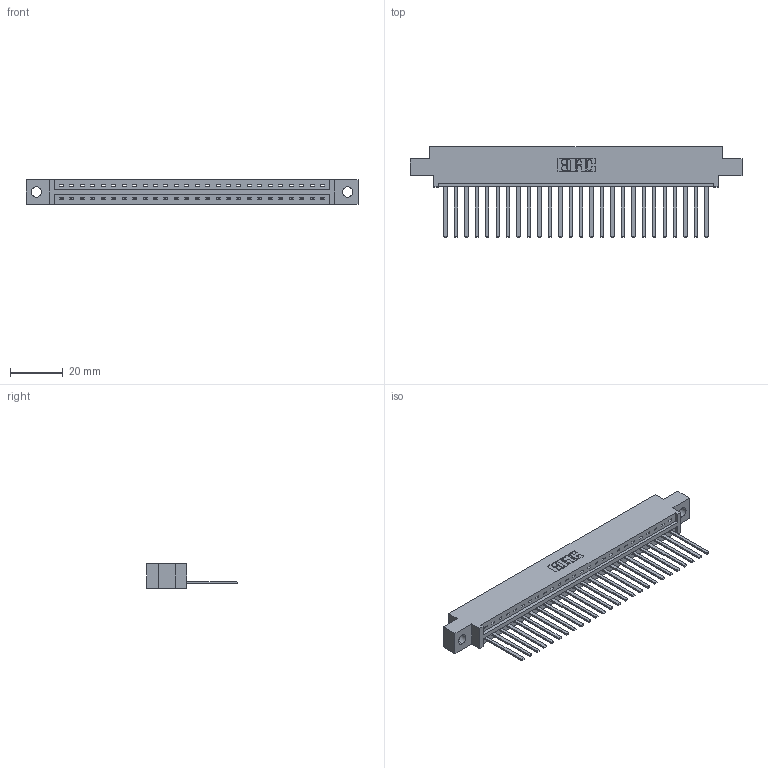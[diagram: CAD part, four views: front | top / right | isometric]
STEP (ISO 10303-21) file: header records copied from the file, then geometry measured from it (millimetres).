
FILE_DESCRIPTION (( 'STEP AP203' ), '1' );
FILE_NAME ('337-026-544-604.STEP', '2019-09-30T19:03:22', ( '' ), ( '' ), 'SwSTEP 2.0', 'SolidWorks 2016', '' );
FILE_SCHEMA (( 'CONFIG_CONTROL_DESIGN' ));
Length unit declared in the file: inch
Products named in the file (3): 337-026-544-604; 345-292-001_345-293-144; 337 Part_0.170 Offset - 0.156 Dia-TH
Assembly tree (27 placements, depth 2):
  337-026-544-604
    337 Part_0.170 Offset - 0.156 Dia-TH
    345-292-001_345-293-144  x26
Bounding box: 126.03 x 34.3 x 9.4 mm (x, y, z)
Volume: 12994.7 mm3; surface area: 14221.6 mm2
Topology: 27 solids, 27 shells, 1574 faces, 4743 edges, 3126 vertices
Faces by surface type: plane 1166, cylinder 408
Entity records: 21347 total; most frequent: CARTESIAN_POINT 3724, ORIENTED_EDGE 3686, DIRECTION 3163, EDGE_CURVE 1843, LINE 1719, VECTOR 1719, VERTEX_POINT 1226, AXIS2_PLACEMENT_3D 722
